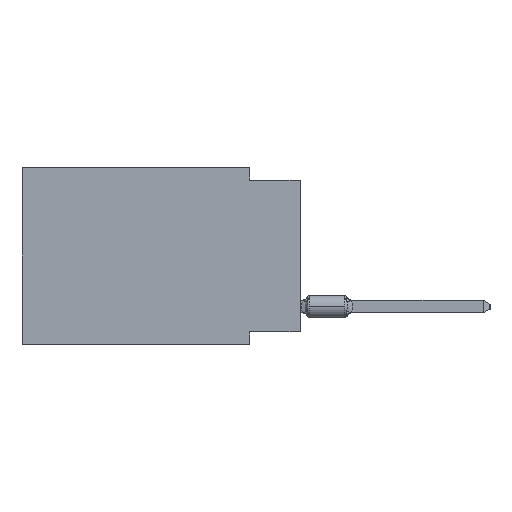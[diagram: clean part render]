
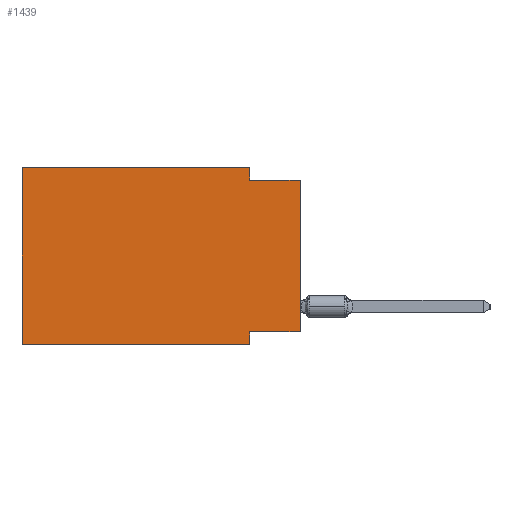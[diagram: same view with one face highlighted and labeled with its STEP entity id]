
A CAD part, left-side view. The second image highlights one B-rep face of the part: STEP entity #1439.
In plain terms, the highlighted planar face has unit normal (-1, 0, 0).
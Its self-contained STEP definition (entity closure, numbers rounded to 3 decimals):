
#355 = CARTESIAN_POINT ( 'NONE',  ( 0., 2.54, 0. ) ) ;
#1146 = VERTEX_POINT ( 'NONE', #28204 ) ;
#1303 = DIRECTION ( 'NONE',  ( 0., 0., -1. ) ) ;
#1439 = ADVANCED_FACE ( 'NONE', ( #26919 ), #29211, .F. ) ;
#2780 = AXIS2_PLACEMENT_3D ( 'NONE', #8448, #6159, #24641 ) ;
#2841 = CARTESIAN_POINT ( 'NONE',  ( 0., 2.54, -0.635 ) ) ;
#3357 = VERTEX_POINT ( 'NONE', #28699 ) ;
#3687 = VECTOR ( 'NONE', #20510, 1000. ) ;
#3867 = VECTOR ( 'NONE', #1303, 1000. ) ;
#4323 = CARTESIAN_POINT ( 'NONE',  ( 0., 2.54, -8.89 ) ) ;
#4501 = LINE ( 'NONE', #27071, #19281 ) ;
#5080 = ORIENTED_EDGE ( 'NONE', *, *, #21290, .F. ) ;
#5334 = LINE ( 'NONE', #355, #18410 ) ;
#5779 = CARTESIAN_POINT ( 'NONE',  ( 0., 13.97, 0. ) ) ;
#6159 = DIRECTION ( 'NONE',  ( 1., 0., 0. ) ) ;
#6426 = EDGE_CURVE ( 'NONE', #1146, #14285, #19764, .T. ) ;
#8448 = CARTESIAN_POINT ( 'NONE',  ( 0., 13.97, 0. ) ) ;
#8746 = ORIENTED_EDGE ( 'NONE', *, *, #10480, .F. ) ;
#9033 = VERTEX_POINT ( 'NONE', #2841 ) ;
#9124 = CARTESIAN_POINT ( 'NONE',  ( 0., 13.97, -8.89 ) ) ;
#9593 = EDGE_CURVE ( 'NONE', #9033, #14285, #4501, .T. ) ;
#9976 = ORIENTED_EDGE ( 'NONE', *, *, #9593, .F. ) ;
#10480 = EDGE_CURVE ( 'NONE', #1146, #13866, #29879, .T. ) ;
#11394 = CARTESIAN_POINT ( 'NONE',  ( 0., 0., -8.255 ) ) ;
#11573 = ORIENTED_EDGE ( 'NONE', *, *, #12878, .T. ) ;
#11658 = ORIENTED_EDGE ( 'NONE', *, *, #26846, .F. ) ;
#11759 = VERTEX_POINT ( 'NONE', #9124 ) ;
#12878 = EDGE_CURVE ( 'NONE', #11759, #3357, #29609, .T. ) ;
#13076 = CARTESIAN_POINT ( 'NONE',  ( 0., 13.97, -8.89 ) ) ;
#13403 = CARTESIAN_POINT ( 'NONE',  ( 0., 0., 0. ) ) ;
#13413 = LINE ( 'NONE', #4323, #3867 ) ;
#13558 = VECTOR ( 'NONE', #26834, 1000. ) ;
#13740 = DIRECTION ( 'NONE',  ( 0., -1., 0. ) ) ;
#13866 = VERTEX_POINT ( 'NONE', #14706 ) ;
#14285 = VERTEX_POINT ( 'NONE', #22198 ) ;
#14579 = DIRECTION ( 'NONE',  ( 0., 0., -1. ) ) ;
#14706 = CARTESIAN_POINT ( 'NONE',  ( 0., 2.54, -8.255 ) ) ;
#15279 = DIRECTION ( 'NONE',  ( 0., 0., 1. ) ) ;
#17035 = VECTOR ( 'NONE', #22652, 1000. ) ;
#17615 = CARTESIAN_POINT ( 'NONE',  ( 0., 13.97, 0. ) ) ;
#17880 = ORIENTED_EDGE ( 'NONE', *, *, #27365, .F. ) ;
#18087 = ORIENTED_EDGE ( 'NONE', *, *, #28929, .F. ) ;
#18410 = VECTOR ( 'NONE', #14579, 1000. ) ;
#19225 = LINE ( 'NONE', #26650, #25208 ) ;
#19281 = VECTOR ( 'NONE', #13740, 1000. ) ;
#19764 = LINE ( 'NONE', #13403, #17035 ) ;
#19978 = VERTEX_POINT ( 'NONE', #17615 ) ;
#20510 = DIRECTION ( 'NONE',  ( 0., -1., 0. ) ) ;
#21290 = EDGE_CURVE ( 'NONE', #19978, #22771, #26692, .T. ) ;
#21379 = CARTESIAN_POINT ( 'NONE',  ( 0., 2.54, 0. ) ) ;
#21653 = EDGE_LOOP ( 'NONE', ( #28374, #9976, #11658, #5080, #17880, #11573, #18087, #8746 ) ) ;
#22198 = CARTESIAN_POINT ( 'NONE',  ( 0., 0., -0.635 ) ) ;
#22652 = DIRECTION ( 'NONE',  ( 0., 0., 1. ) ) ;
#22771 = VERTEX_POINT ( 'NONE', #21379 ) ;
#23363 = DIRECTION ( 'NONE',  ( 0., 1., 0. ) ) ;
#24641 = DIRECTION ( 'NONE',  ( 0., 0., -1. ) ) ;
#25208 = VECTOR ( 'NONE', #15279, 1000. ) ;
#26650 = CARTESIAN_POINT ( 'NONE',  ( 0., 13.97, 0. ) ) ;
#26692 = LINE ( 'NONE', #5779, #13558 ) ;
#26834 = DIRECTION ( 'NONE',  ( 0., -1., 0. ) ) ;
#26846 = EDGE_CURVE ( 'NONE', #22771, #9033, #5334, .T. ) ;
#26919 = FACE_OUTER_BOUND ( 'NONE', #21653, .T. ) ;
#27071 = CARTESIAN_POINT ( 'NONE',  ( 0., 0., -0.635 ) ) ;
#27365 = EDGE_CURVE ( 'NONE', #11759, #19978, #19225, .T. ) ;
#28204 = CARTESIAN_POINT ( 'NONE',  ( 0., 0., -8.255 ) ) ;
#28374 = ORIENTED_EDGE ( 'NONE', *, *, #6426, .T. ) ;
#28699 = CARTESIAN_POINT ( 'NONE',  ( 0., 2.54, -8.89 ) ) ;
#28929 = EDGE_CURVE ( 'NONE', #13866, #3357, #13413, .T. ) ;
#29211 = PLANE ( 'NONE',  #2780 ) ;
#29609 = LINE ( 'NONE', #13076, #3687 ) ;
#29879 = LINE ( 'NONE', #11394, #29948 ) ;
#29948 = VECTOR ( 'NONE', #23363, 1000. ) ;
